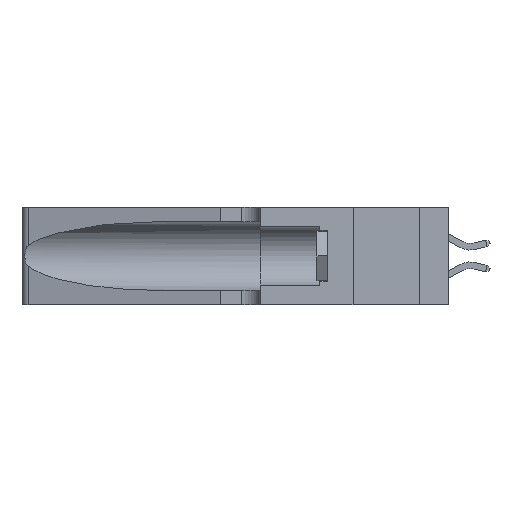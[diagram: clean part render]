
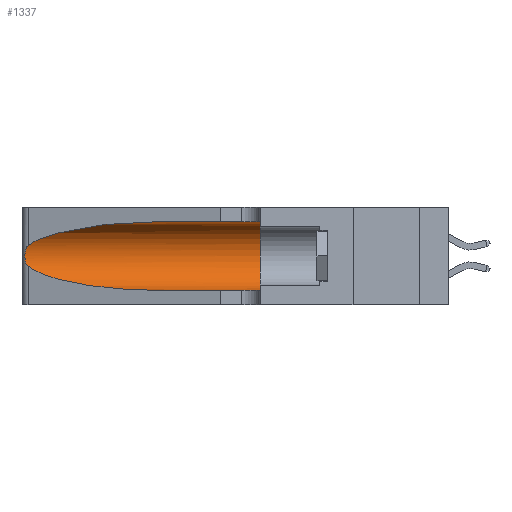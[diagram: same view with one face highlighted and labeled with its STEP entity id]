
A CAD part, left-side view. The second image highlights one B-rep face of the part: STEP entity #1337.
In plain terms, the highlighted cylindrical face has radius 3.308 mm (diameter 6.617 mm), a partial arc.
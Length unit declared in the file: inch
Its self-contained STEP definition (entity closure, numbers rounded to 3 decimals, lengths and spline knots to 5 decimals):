
#80 =( BOUNDED_CURVE ( )  B_SPLINE_CURVE ( 3, ( #19176, #203, #1683, #11316 ),
 .UNSPECIFIED., .F., .F. ) 
 B_SPLINE_CURVE_WITH_KNOTS ( ( 4, 4 ),
 ( 1.5708, 2.84003 ),
 .UNSPECIFIED. ) 
 CURVE ( )  GEOMETRIC_REPRESENTATION_ITEM ( )  RATIONAL_B_SPLINE_CURVE ( ( 1., 0.87, 0.87, 1. ) ) 
 REPRESENTATION_ITEM ( '' )  );
#136 = LINE ( 'NONE', #11604, #2884 ) ;
#203 = CARTESIAN_POINT ( 'NONE',  ( 0.18966, 0.96281, 0.31525 ) ) ;
#1337 = ADVANCED_FACE ( 'NONE', ( #19174 ), #10281, .F. ) ;
#1648 = ORIENTED_EDGE ( 'NONE', *, *, #2849, .F. ) ;
#1683 = CARTESIAN_POINT ( 'NONE',  ( 0.2373, 1.15595, 0.28018 ) ) ;
#2413 = CARTESIAN_POINT ( 'NONE',  ( 0.25854, 1.2359, 0.20912 ) ) ;
#2666 = CARTESIAN_POINT ( 'NONE',  ( 0.26075, 1.23896, 0.178 ) ) ;
#2849 = EDGE_CURVE ( 'NONE', #12182, #11910, #17220, .T. ) ;
#2884 = VECTOR ( 'NONE', #5471, 39.37008 ) ;
#3925 = CARTESIAN_POINT ( 'NONE',  ( 0.25487, 1.22718, 0.14631 ) ) ;
#5144 = ORIENTED_EDGE ( 'NONE', *, *, #18671, .T. ) ;
#5305 = DIRECTION ( 'NONE',  ( 0., -1., 0. ) ) ;
#5471 = DIRECTION ( 'NONE',  ( 0., -1., 0. ) ) ;
#5661 = CARTESIAN_POINT ( 'NONE',  ( 0.1305, 0.72297, 0.31525 ) ) ;
#6186 = EDGE_CURVE ( 'NONE', #17125, #18219, #14178, .T. ) ;
#6191 = CARTESIAN_POINT ( 'NONE',  ( 0.1305, 0.72297, 0.05475 ) ) ;
#6864 = CARTESIAN_POINT ( 'NONE',  ( 0.25639, 1.23186, 0.15144 ) ) ;
#7126 = EDGE_CURVE ( 'NONE', #12182, #17125, #80, .T. ) ;
#7712 = AXIS2_PLACEMENT_3D ( 'NONE', #11358, #5305, #19442 ) ;
#8286 = VECTOR ( 'NONE', #14693, 39.37008 ) ;
#8594 = CARTESIAN_POINT ( 'NONE',  ( 0.25555, 1.22994, 0.2215 ) ) ;
#9001 =( BOUNDED_CURVE ( )  B_SPLINE_CURVE ( 3, ( #20084, #12540, #12738, #6191 ),
 .UNSPECIFIED., .F., .T. ) 
 B_SPLINE_CURVE_WITH_KNOTS ( ( 4, 4 ),
 ( 3.44316, 4.71239 ),
 .UNSPECIFIED. ) 
 CURVE ( )  GEOMETRIC_REPRESENTATION_ITEM ( )  RATIONAL_B_SPLINE_CURVE ( ( 1., 0.87, 0.87, 1. ) ) 
 REPRESENTATION_ITEM ( '' )  );
#9655 = EDGE_LOOP ( 'NONE', ( #16916, #11040, #13534, #5144, #16100, #1648 ) ) ;
#9946 = EDGE_CURVE ( 'NONE', #18219, #13302, #9001, .T. ) ;
#10253 = CARTESIAN_POINT ( 'NONE',  ( 0.25487, 1.22718, 0.22369 ) ) ;
#10281 = CYLINDRICAL_SURFACE ( 'NONE', #7712, 0.13025 ) ;
#10386 = CARTESIAN_POINT ( 'NONE',  ( 0.26075, 1.23896, 0.19203 ) ) ;
#10494 = DIRECTION ( 'NONE',  ( 0., 1., 0. ) ) ;
#11040 = ORIENTED_EDGE ( 'NONE', *, *, #6186, .T. ) ;
#11316 = CARTESIAN_POINT ( 'NONE',  ( 0.25487, 1.22718, 0.22369 ) ) ;
#11358 = CARTESIAN_POINT ( 'NONE',  ( 0.1305, 1.61858, 0.185 ) ) ;
#11474 = CARTESIAN_POINT ( 'NONE',  ( 0.25487, 1.22718, 0.14631 ) ) ;
#11604 = CARTESIAN_POINT ( 'NONE',  ( 0.1305, 1.61858, 0.05475 ) ) ;
#11676 = CARTESIAN_POINT ( 'NONE',  ( 0.25856, 1.23593, 0.16098 ) ) ;
#11806 = AXIS2_PLACEMENT_3D ( 'NONE', #14680, #10494, #12076 ) ;
#11840 = CARTESIAN_POINT ( 'NONE',  ( 0.25639, 1.23184, 0.21858 ) ) ;
#11910 = VERTEX_POINT ( 'NONE', #14530 ) ;
#12076 = DIRECTION ( 'NONE',  ( 0., 0., 1. ) ) ;
#12182 = VERTEX_POINT ( 'NONE', #5661 ) ;
#12540 = CARTESIAN_POINT ( 'NONE',  ( 0.2373, 1.15595, 0.08982 ) ) ;
#12738 = CARTESIAN_POINT ( 'NONE',  ( 0.18966, 0.96281, 0.05475 ) ) ;
#13302 = VERTEX_POINT ( 'NONE', #19127 ) ;
#13506 = VERTEX_POINT ( 'NONE', #13565 ) ;
#13534 = ORIENTED_EDGE ( 'NONE', *, *, #9946, .T. ) ;
#13565 = CARTESIAN_POINT ( 'NONE',  ( 0.1305, 0.35, 0.05475 ) ) ;
#14178 = B_SPLINE_CURVE_WITH_KNOTS ( 'NONE', 3,
 ( #10253, #8594, #11840, #16571, #2413, #15053, #10386, #2666, #16346, #11676, #17854, #6864, #17993, #11474 ),
 .UNSPECIFIED., .F., .F.,
 ( 4, 2, 2, 2, 2, 2, 4 ),
 ( 0., 0.00027, 0.00053, 0.00107, 0.0016, 0.00187, 0.00214 ),
 .UNSPECIFIED. ) ;
#14466 = CARTESIAN_POINT ( 'NONE',  ( 0.25487, 1.22718, 0.22369 ) ) ;
#14530 = CARTESIAN_POINT ( 'NONE',  ( 0.1305, 0.35, 0.31525 ) ) ;
#14680 = CARTESIAN_POINT ( 'NONE',  ( 0.1305, 0.35, 0.185 ) ) ;
#14693 = DIRECTION ( 'NONE',  ( 0., -1., 0. ) ) ;
#15053 = CARTESIAN_POINT ( 'NONE',  ( 0.26018, 1.23835, 0.19895 ) ) ;
#15188 = CARTESIAN_POINT ( 'NONE',  ( 0.1305, 1.61858, 0.31525 ) ) ;
#16100 = ORIENTED_EDGE ( 'NONE', *, *, #18674, .F. ) ;
#16223 = CIRCLE ( 'NONE', #11806, 0.13025 ) ;
#16346 = CARTESIAN_POINT ( 'NONE',  ( 0.26017, 1.23833, 0.17102 ) ) ;
#16571 = CARTESIAN_POINT ( 'NONE',  ( 0.25787, 1.23484, 0.2124 ) ) ;
#16916 = ORIENTED_EDGE ( 'NONE', *, *, #7126, .T. ) ;
#17125 = VERTEX_POINT ( 'NONE', #14466 ) ;
#17220 = LINE ( 'NONE', #15188, #8286 ) ;
#17854 = CARTESIAN_POINT ( 'NONE',  ( 0.25789, 1.23486, 0.15765 ) ) ;
#17993 = CARTESIAN_POINT ( 'NONE',  ( 0.25555, 1.22993, 0.14849 ) ) ;
#18219 = VERTEX_POINT ( 'NONE', #3925 ) ;
#18671 = EDGE_CURVE ( 'NONE', #13302, #13506, #136, .T. ) ;
#18674 = EDGE_CURVE ( 'NONE', #11910, #13506, #16223, .T. ) ;
#19127 = CARTESIAN_POINT ( 'NONE',  ( 0.1305, 0.72297, 0.05475 ) ) ;
#19174 = FACE_OUTER_BOUND ( 'NONE', #9655, .T. ) ;
#19176 = CARTESIAN_POINT ( 'NONE',  ( 0.1305, 0.72297, 0.31525 ) ) ;
#19442 = DIRECTION ( 'NONE',  ( 0., 0., -1. ) ) ;
#20084 = CARTESIAN_POINT ( 'NONE',  ( 0.25487, 1.22718, 0.14631 ) ) ;
